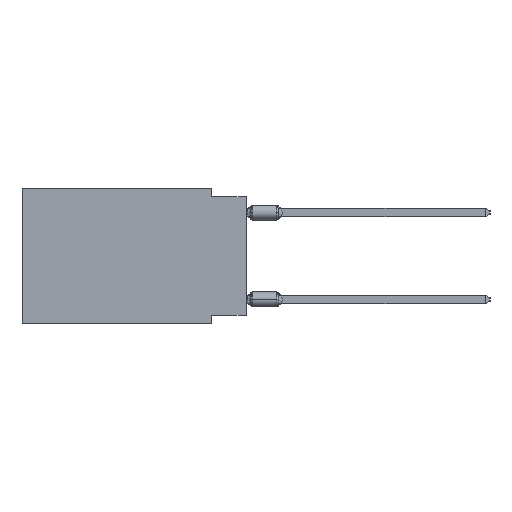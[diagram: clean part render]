
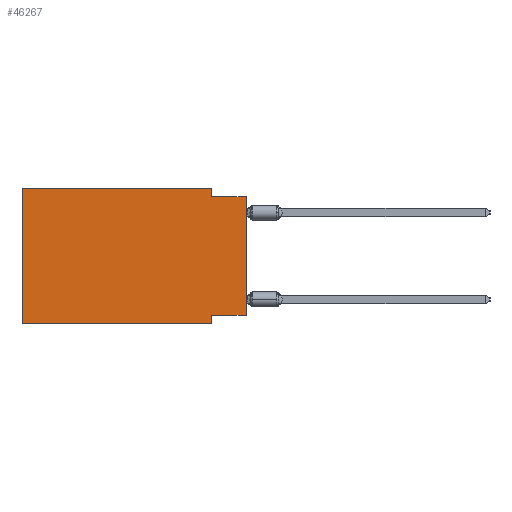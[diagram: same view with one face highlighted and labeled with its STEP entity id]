
A CAD part, left-side view. The second image highlights one B-rep face of the part: STEP entity #46267.
In plain terms, the highlighted planar face has unit normal (-1, 0, 0).
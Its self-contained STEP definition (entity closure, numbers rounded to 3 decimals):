
#260 = VECTOR ( 'NONE', #13955, 1000. ) ;
#332 = VECTOR ( 'NONE', #17396, 1000. ) ;
#1083 = ORIENTED_EDGE ( 'NONE', *, *, #20726, .F. ) ;
#1479 = EDGE_CURVE ( 'NONE', #18711, #44592, #29956, .T. ) ;
#3110 = CARTESIAN_POINT ( 'NONE',  ( 0., 2.54, 0. ) ) ;
#3216 = ORIENTED_EDGE ( 'NONE', *, *, #9183, .T. ) ;
#3546 = PLANE ( 'NONE',  #15459 ) ;
#3872 = ORIENTED_EDGE ( 'NONE', *, *, #38746, .F. ) ;
#7394 = EDGE_CURVE ( 'NONE', #23166, #33387, #33472, .T. ) ;
#8126 = EDGE_CURVE ( 'NONE', #33387, #22160, #47560, .T. ) ;
#9183 = EDGE_CURVE ( 'NONE', #23166, #44512, #47231, .T. ) ;
#10333 = CARTESIAN_POINT ( 'NONE',  ( 0., 2.54, 0. ) ) ;
#10450 = CARTESIAN_POINT ( 'NONE',  ( 0., 16.383, 0. ) ) ;
#10612 = ORIENTED_EDGE ( 'NONE', *, *, #7394, .F. ) ;
#10958 = CARTESIAN_POINT ( 'NONE',  ( 0., 16.383, 0. ) ) ;
#11235 = EDGE_CURVE ( 'NONE', #13855, #34998, #29845, .T. ) ;
#11524 = DIRECTION ( 'NONE',  ( 0., 0., -1. ) ) ;
#12987 = CARTESIAN_POINT ( 'NONE',  ( 0., 0., 0. ) ) ;
#13556 = DIRECTION ( 'NONE',  ( 0., 0., -1. ) ) ;
#13855 = VERTEX_POINT ( 'NONE', #10333 ) ;
#13888 = LINE ( 'NONE', #24655, #332 ) ;
#13955 = DIRECTION ( 'NONE',  ( 0., -1., 0. ) ) ;
#14465 = DIRECTION ( 'NONE',  ( 0., 1., 0. ) ) ;
#15459 = AXIS2_PLACEMENT_3D ( 'NONE', #18794, #34039, #11524 ) ;
#16357 = ORIENTED_EDGE ( 'NONE', *, *, #1479, .F. ) ;
#17396 = DIRECTION ( 'NONE',  ( 0., -1., 0. ) ) ;
#18463 = DIRECTION ( 'NONE',  ( 0., 0., 1. ) ) ;
#18711 = VERTEX_POINT ( 'NONE', #28201 ) ;
#18794 = CARTESIAN_POINT ( 'NONE',  ( 0., 16.383, 0. ) ) ;
#19469 = CARTESIAN_POINT ( 'NONE',  ( 0., 2.54, -0.635 ) ) ;
#20726 = EDGE_CURVE ( 'NONE', #34998, #44512, #13888, .T. ) ;
#21240 = VECTOR ( 'NONE', #14465, 1000. ) ;
#21936 = DIRECTION ( 'NONE',  ( 0., -1., 0. ) ) ;
#22160 = VERTEX_POINT ( 'NONE', #30686 ) ;
#22721 = CARTESIAN_POINT ( 'NONE',  ( 0., 0., -9.271 ) ) ;
#23166 = VERTEX_POINT ( 'NONE', #24231 ) ;
#23820 = ORIENTED_EDGE ( 'NONE', *, *, #8126, .F. ) ;
#24231 = CARTESIAN_POINT ( 'NONE',  ( 0., 0., -9.271 ) ) ;
#24417 = ORIENTED_EDGE ( 'NONE', *, *, #35215, .T. ) ;
#24655 = CARTESIAN_POINT ( 'NONE',  ( 0., 0., -0.635 ) ) ;
#26219 = DIRECTION ( 'NONE',  ( 0., 0., 1. ) ) ;
#27068 = CARTESIAN_POINT ( 'NONE',  ( 0., 0., -0.635 ) ) ;
#28201 = CARTESIAN_POINT ( 'NONE',  ( 0., 16.383, -9.906 ) ) ;
#29590 = DIRECTION ( 'NONE',  ( 0., 0., -1. ) ) ;
#29675 = LINE ( 'NONE', #10450, #260 ) ;
#29845 = LINE ( 'NONE', #3110, #37441 ) ;
#29956 = LINE ( 'NONE', #10958, #36826 ) ;
#30077 = CARTESIAN_POINT ( 'NONE',  ( 0., 16.383, 0. ) ) ;
#30686 = CARTESIAN_POINT ( 'NONE',  ( 0., 2.54, -9.906 ) ) ;
#33387 = VERTEX_POINT ( 'NONE', #34034 ) ;
#33472 = LINE ( 'NONE', #22721, #21240 ) ;
#34034 = CARTESIAN_POINT ( 'NONE',  ( 0., 2.54, -9.271 ) ) ;
#34039 = DIRECTION ( 'NONE',  ( 1., 0., 0. ) ) ;
#34111 = ORIENTED_EDGE ( 'NONE', *, *, #11235, .F. ) ;
#34998 = VERTEX_POINT ( 'NONE', #19469 ) ;
#35215 = EDGE_CURVE ( 'NONE', #18711, #22160, #44921, .T. ) ;
#36308 = CARTESIAN_POINT ( 'NONE',  ( 0., 2.54, -9.906 ) ) ;
#36764 = VECTOR ( 'NONE', #21936, 1000. ) ;
#36826 = VECTOR ( 'NONE', #26219, 1000. ) ;
#37169 = CARTESIAN_POINT ( 'NONE',  ( 0., 16.383, -9.906 ) ) ;
#37255 = VECTOR ( 'NONE', #13556, 1000. ) ;
#37441 = VECTOR ( 'NONE', #29590, 1000. ) ;
#37770 = FACE_OUTER_BOUND ( 'NONE', #38144, .T. ) ;
#38116 = VECTOR ( 'NONE', #18463, 1000. ) ;
#38144 = EDGE_LOOP ( 'NONE', ( #3216, #1083, #34111, #3872, #16357, #24417, #23820, #10612 ) ) ;
#38746 = EDGE_CURVE ( 'NONE', #44592, #13855, #29675, .T. ) ;
#44512 = VERTEX_POINT ( 'NONE', #27068 ) ;
#44592 = VERTEX_POINT ( 'NONE', #30077 ) ;
#44921 = LINE ( 'NONE', #37169, #36764 ) ;
#46267 = ADVANCED_FACE ( 'NONE', ( #37770 ), #3546, .F. ) ;
#47231 = LINE ( 'NONE', #12987, #38116 ) ;
#47560 = LINE ( 'NONE', #36308, #37255 ) ;
